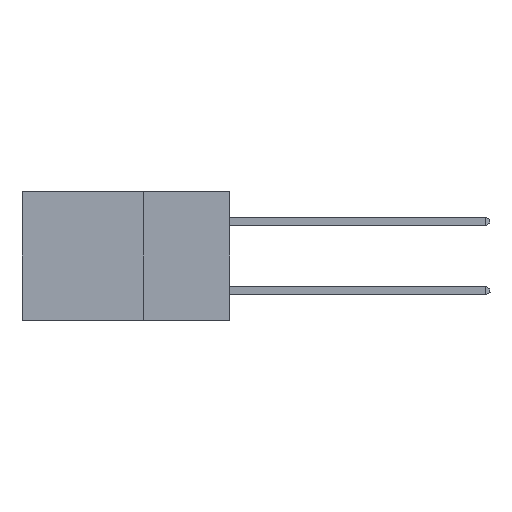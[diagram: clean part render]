
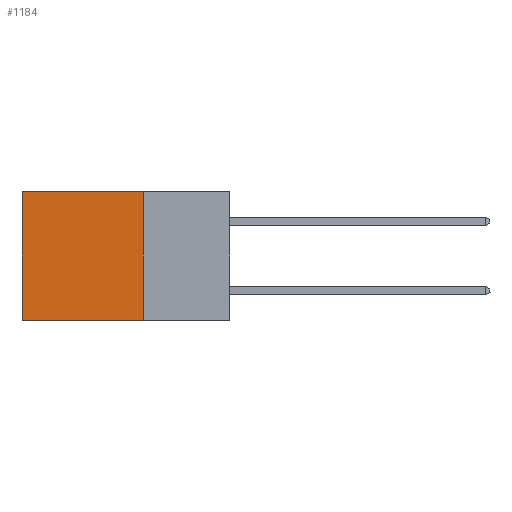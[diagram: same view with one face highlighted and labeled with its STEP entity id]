
A CAD part, left-side view. The second image highlights one B-rep face of the part: STEP entity #1184.
In plain terms, the highlighted planar face has unit normal (-1, 0, 0).
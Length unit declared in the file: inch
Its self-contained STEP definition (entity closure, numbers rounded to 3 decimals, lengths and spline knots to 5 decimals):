
#178 = ORIENTED_EDGE ( 'NONE', *, *, #12920, .F. ) ;
#282 = CARTESIAN_POINT ( 'NONE',  ( 0.298, 0.25, -0.37 ) ) ;
#303 = DIRECTION ( 'NONE',  ( 0., 0., -1. ) ) ;
#460 = EDGE_CURVE ( 'NONE', #9691, #9171, #8916, .T. ) ;
#708 = AXIS2_PLACEMENT_3D ( 'NONE', #9367, #8088, #12944 ) ;
#1184 = ADVANCED_FACE ( 'NONE', ( #13240 ), #11846, .F. ) ;
#1315 = LINE ( 'NONE', #5301, #3867 ) ;
#1408 = CARTESIAN_POINT ( 'NONE',  ( 0.298, 0.25, -0.37 ) ) ;
#3253 = ORIENTED_EDGE ( 'NONE', *, *, #13671, .T. ) ;
#3867 = VECTOR ( 'NONE', #303, 39.37008 ) ;
#3908 = DIRECTION ( 'NONE',  ( 0., 0., -1. ) ) ;
#4266 = VERTEX_POINT ( 'NONE', #8727 ) ;
#4288 = CARTESIAN_POINT ( 'NONE',  ( 0.298, 0.6, -0.37 ) ) ;
#4747 = EDGE_CURVE ( 'NONE', #4266, #9263, #11949, .T. ) ;
#5301 = CARTESIAN_POINT ( 'NONE',  ( 0.298, 0.25, 0. ) ) ;
#5603 = VECTOR ( 'NONE', #11893, 39.37008 ) ;
#7011 = VECTOR ( 'NONE', #3908, 39.37008 ) ;
#8088 = DIRECTION ( 'NONE',  ( 1., 0., 0. ) ) ;
#8245 = EDGE_LOOP ( 'NONE', ( #3253, #16046, #178, #12366 ) ) ;
#8727 = CARTESIAN_POINT ( 'NONE',  ( 0.298, 0.25, 0. ) ) ;
#8916 = LINE ( 'NONE', #282, #11097 ) ;
#9171 = VERTEX_POINT ( 'NONE', #4288 ) ;
#9263 = VERTEX_POINT ( 'NONE', #12110 ) ;
#9367 = CARTESIAN_POINT ( 'NONE',  ( 0.298, 0.25, 0. ) ) ;
#9691 = VERTEX_POINT ( 'NONE', #1408 ) ;
#10427 = DIRECTION ( 'NONE',  ( 0., 1., 0. ) ) ;
#11097 = VECTOR ( 'NONE', #10427, 39.37008 ) ;
#11846 = PLANE ( 'NONE',  #708 ) ;
#11893 = DIRECTION ( 'NONE',  ( 0., 1., 0. ) ) ;
#11949 = LINE ( 'NONE', #14200, #5603 ) ;
#12110 = CARTESIAN_POINT ( 'NONE',  ( 0.298, 0.6, 0. ) ) ;
#12366 = ORIENTED_EDGE ( 'NONE', *, *, #4747, .T. ) ;
#12603 = CARTESIAN_POINT ( 'NONE',  ( 0.298, 0.6, 0. ) ) ;
#12920 = EDGE_CURVE ( 'NONE', #4266, #9691, #1315, .T. ) ;
#12944 = DIRECTION ( 'NONE',  ( 0., 0., -1. ) ) ;
#12946 = LINE ( 'NONE', #12603, #7011 ) ;
#13240 = FACE_OUTER_BOUND ( 'NONE', #8245, .T. ) ;
#13671 = EDGE_CURVE ( 'NONE', #9263, #9171, #12946, .T. ) ;
#14200 = CARTESIAN_POINT ( 'NONE',  ( 0.298, 0.25, 0. ) ) ;
#16046 = ORIENTED_EDGE ( 'NONE', *, *, #460, .F. ) ;
